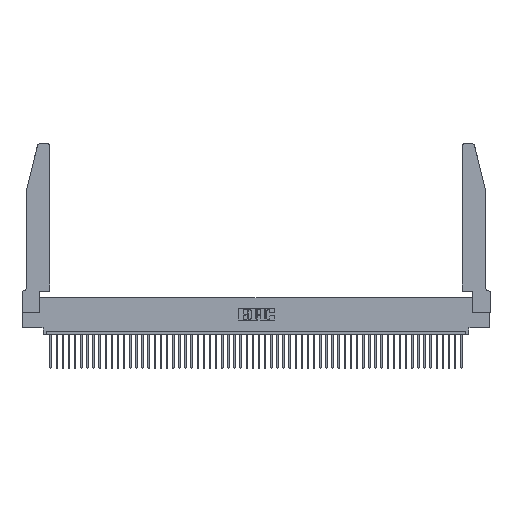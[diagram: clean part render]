
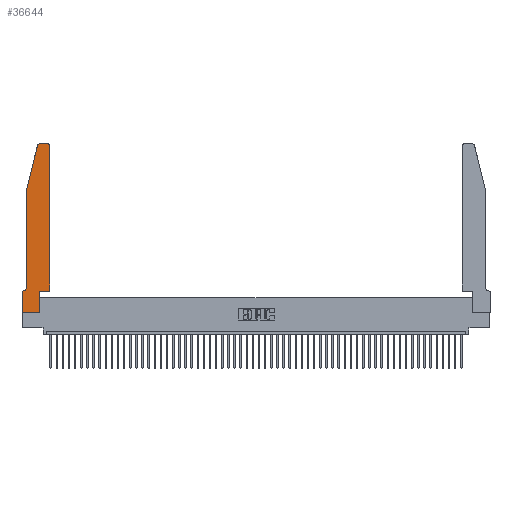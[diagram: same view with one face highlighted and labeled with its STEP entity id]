
A CAD part, top view. The second image highlights one B-rep face of the part: STEP entity #36644.
In plain terms, the highlighted planar face has unit normal (0, 0, 1).
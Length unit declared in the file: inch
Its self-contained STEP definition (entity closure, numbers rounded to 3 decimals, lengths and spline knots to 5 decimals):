
#711 = DIRECTION ( 'NONE',  ( 1., 0., 0. ) ) ;
#966 = LINE ( 'NONE', #21092, #16319 ) ;
#1017 = ORIENTED_EDGE ( 'NONE', *, *, #37235, .T. ) ;
#1078 = ORIENTED_EDGE ( 'NONE', *, *, #22774, .T. ) ;
#1677 = AXIS2_PLACEMENT_3D ( 'NONE', #40886, #33396, #37503 ) ;
#1744 = LINE ( 'NONE', #2348, #32974 ) ;
#1917 = DIRECTION ( 'NONE',  ( 1., 0., 0. ) ) ;
#2348 = CARTESIAN_POINT ( 'NONE',  ( 0.4505, 0.35, 0.37 ) ) ;
#2790 = VECTOR ( 'NONE', #35138, 39.37008 ) ;
#3698 = ORIENTED_EDGE ( 'NONE', *, *, #28009, .T. ) ;
#4113 = VERTEX_POINT ( 'NONE', #11227 ) ;
#4486 = DIRECTION ( 'NONE',  ( 0., 1., 0. ) ) ;
#4513 = CARTESIAN_POINT ( 'NONE',  ( 0.0755, 0.35, 0.37 ) ) ;
#4960 = EDGE_CURVE ( 'NONE', #20387, #7002, #966, .T. ) ;
#5145 = VERTEX_POINT ( 'NONE', #26434 ) ;
#5628 = CARTESIAN_POINT ( 'NONE',  ( 0., 0., 0.37 ) ) ;
#5885 = CARTESIAN_POINT ( 'NONE',  ( 0.4505, 0.35, 0.37 ) ) ;
#6664 = EDGE_CURVE ( 'NONE', #32335, #20387, #12379, .T. ) ;
#7002 = VERTEX_POINT ( 'NONE', #29811 ) ;
#7360 = CARTESIAN_POINT ( 'NONE',  ( 0.284, 2.75, 0.37 ) ) ;
#7570 = CARTESIAN_POINT ( 'NONE',  ( 0.4205, 2.75, 0.37 ) ) ;
#8234 = ORIENTED_EDGE ( 'NONE', *, *, #17785, .T. ) ;
#8280 = VERTEX_POINT ( 'NONE', #37958 ) ;
#10354 = EDGE_LOOP ( 'NONE', ( #41073, #41294, #10816, #1078, #29837, #8234, #47547, #3698, #49440, #22198, #49227, #1017 ) ) ;
#10816 = ORIENTED_EDGE ( 'NONE', *, *, #4960, .T. ) ;
#11107 = CARTESIAN_POINT ( 'NONE',  ( 0., 0.35, 0.37 ) ) ;
#11115 = EDGE_CURVE ( 'NONE', #13756, #30331, #36003, .T. ) ;
#11186 = VECTOR ( 'NONE', #1917, 39.37008 ) ;
#11227 = CARTESIAN_POINT ( 'NONE',  ( 0., 0., 0.37 ) ) ;
#12379 = CIRCLE ( 'NONE', #46771, 0.03 ) ;
#13756 = VERTEX_POINT ( 'NONE', #23591 ) ;
#13993 = CARTESIAN_POINT ( 'NONE',  ( 0.4505, 0.35, 0.37 ) ) ;
#16002 = CARTESIAN_POINT ( 'NONE',  ( 0.4205, 2.72, 0.37 ) ) ;
#16081 = CARTESIAN_POINT ( 'NONE',  ( 0.0755, 0.42, 0.37 ) ) ;
#16158 = DIRECTION ( 'NONE',  ( 0., 0., 1. ) ) ;
#16319 = VECTOR ( 'NONE', #25358, 39.37008 ) ;
#17333 = LINE ( 'NONE', #36458, #52323 ) ;
#17785 = EDGE_CURVE ( 'NONE', #5145, #8280, #45008, .T. ) ;
#18585 = VECTOR ( 'NONE', #49139, 39.37008 ) ;
#19628 = DIRECTION ( 'NONE',  ( 0., 0., 1. ) ) ;
#20029 = CARTESIAN_POINT ( 'NONE',  ( 0.2865, 0., 0.37 ) ) ;
#20387 = VERTEX_POINT ( 'NONE', #51541 ) ;
#21092 = CARTESIAN_POINT ( 'NONE',  ( 0.0755, 2., 0.37 ) ) ;
#21106 = AXIS2_PLACEMENT_3D ( 'NONE', #11107, #19628, #27269 ) ;
#21149 = LINE ( 'NONE', #32936, #51008 ) ;
#21228 = EDGE_CURVE ( 'NONE', #29095, #13756, #21149, .T. ) ;
#22198 = ORIENTED_EDGE ( 'NONE', *, *, #11115, .T. ) ;
#22666 = CIRCLE ( 'NONE', #1677, 0.07 ) ;
#22774 = EDGE_CURVE ( 'NONE', #7002, #44008, #30775, .T. ) ;
#23195 = CARTESIAN_POINT ( 'NONE',  ( 0.4505, 2.72, 0.37 ) ) ;
#23591 = CARTESIAN_POINT ( 'NONE',  ( 0.2865, 0.35, 0.37 ) ) ;
#25358 = DIRECTION ( 'NONE',  ( -0.239, -0.971, 0. ) ) ;
#26434 = CARTESIAN_POINT ( 'NONE',  ( 0.0055, 0.35, 0.37 ) ) ;
#26467 = EDGE_CURVE ( 'NONE', #44008, #5145, #22666, .T. ) ;
#27269 = DIRECTION ( 'NONE',  ( 1., 0., 0. ) ) ;
#28009 = EDGE_CURVE ( 'NONE', #4113, #29095, #29485, .T. ) ;
#28677 = EDGE_CURVE ( 'NONE', #8280, #4113, #29381, .T. ) ;
#29095 = VERTEX_POINT ( 'NONE', #20029 ) ;
#29381 = LINE ( 'NONE', #40776, #18585 ) ;
#29383 = DIRECTION ( 'NONE',  ( -1., 0., 0. ) ) ;
#29485 = LINE ( 'NONE', #5628, #2790 ) ;
#29811 = CARTESIAN_POINT ( 'NONE',  ( 0.0755, 2., 0.37 ) ) ;
#29837 = ORIENTED_EDGE ( 'NONE', *, *, #26467, .T. ) ;
#30331 = VERTEX_POINT ( 'NONE', #5885 ) ;
#30775 = LINE ( 'NONE', #41610, #51897 ) ;
#31661 = EDGE_CURVE ( 'NONE', #34098, #32335, #17333, .T. ) ;
#32335 = VERTEX_POINT ( 'NONE', #7360 ) ;
#32936 = CARTESIAN_POINT ( 'NONE',  ( 0.2865, 0.35, 0.37 ) ) ;
#32974 = VECTOR ( 'NONE', #43419, 39.37008 ) ;
#33336 = CARTESIAN_POINT ( 'NONE',  ( 0.284, 2.72, 0.37 ) ) ;
#33396 = DIRECTION ( 'NONE',  ( 0., 0., -1. ) ) ;
#34098 = VERTEX_POINT ( 'NONE', #7570 ) ;
#34225 = VECTOR ( 'NONE', #29383, 39.37008 ) ;
#35138 = DIRECTION ( 'NONE',  ( 1., 0., 0. ) ) ;
#36003 = LINE ( 'NONE', #13993, #11186 ) ;
#36305 = FACE_OUTER_BOUND ( 'NONE', #10354, .T. ) ;
#36458 = CARTESIAN_POINT ( 'NONE',  ( 0.2605, 2.75, 0.37 ) ) ;
#36644 = ADVANCED_FACE ( 'NONE', ( #36305 ), #43977, .T. ) ;
#37235 = EDGE_CURVE ( 'NONE', #51395, #34098, #38727, .T. ) ;
#37503 = DIRECTION ( 'NONE',  ( -1., 0., 0. ) ) ;
#37958 = CARTESIAN_POINT ( 'NONE',  ( 0., 0.35, 0.37 ) ) ;
#38727 = CIRCLE ( 'NONE', #41193, 0.03 ) ;
#40776 = CARTESIAN_POINT ( 'NONE',  ( 0., 0., 0.37 ) ) ;
#40886 = CARTESIAN_POINT ( 'NONE',  ( 0.0055, 0.42, 0.37 ) ) ;
#41073 = ORIENTED_EDGE ( 'NONE', *, *, #31661, .T. ) ;
#41193 = AXIS2_PLACEMENT_3D ( 'NONE', #16002, #16158, #48459 ) ;
#41294 = ORIENTED_EDGE ( 'NONE', *, *, #6664, .T. ) ;
#41610 = CARTESIAN_POINT ( 'NONE',  ( 0.0755, 2., 0.37 ) ) ;
#43419 = DIRECTION ( 'NONE',  ( 0., 1., 0. ) ) ;
#43977 = PLANE ( 'NONE',  #21106 ) ;
#44008 = VERTEX_POINT ( 'NONE', #16081 ) ;
#45008 = LINE ( 'NONE', #4513, #34225 ) ;
#46018 = DIRECTION ( 'NONE',  ( 0., -1., 0. ) ) ;
#46771 = AXIS2_PLACEMENT_3D ( 'NONE', #33336, #50099, #711 ) ;
#47547 = ORIENTED_EDGE ( 'NONE', *, *, #28677, .T. ) ;
#47760 = DIRECTION ( 'NONE',  ( -1., 0., 0. ) ) ;
#48007 = EDGE_CURVE ( 'NONE', #30331, #51395, #1744, .T. ) ;
#48459 = DIRECTION ( 'NONE',  ( 1., 0., 0. ) ) ;
#49139 = DIRECTION ( 'NONE',  ( 0., -1., 0. ) ) ;
#49227 = ORIENTED_EDGE ( 'NONE', *, *, #48007, .T. ) ;
#49440 = ORIENTED_EDGE ( 'NONE', *, *, #21228, .T. ) ;
#50099 = DIRECTION ( 'NONE',  ( 0., 0., 1. ) ) ;
#51008 = VECTOR ( 'NONE', #4486, 39.37008 ) ;
#51395 = VERTEX_POINT ( 'NONE', #23195 ) ;
#51541 = CARTESIAN_POINT ( 'NONE',  ( 0.25487, 2.72718, 0.37 ) ) ;
#51897 = VECTOR ( 'NONE', #46018, 39.37008 ) ;
#52323 = VECTOR ( 'NONE', #47760, 39.37008 ) ;
